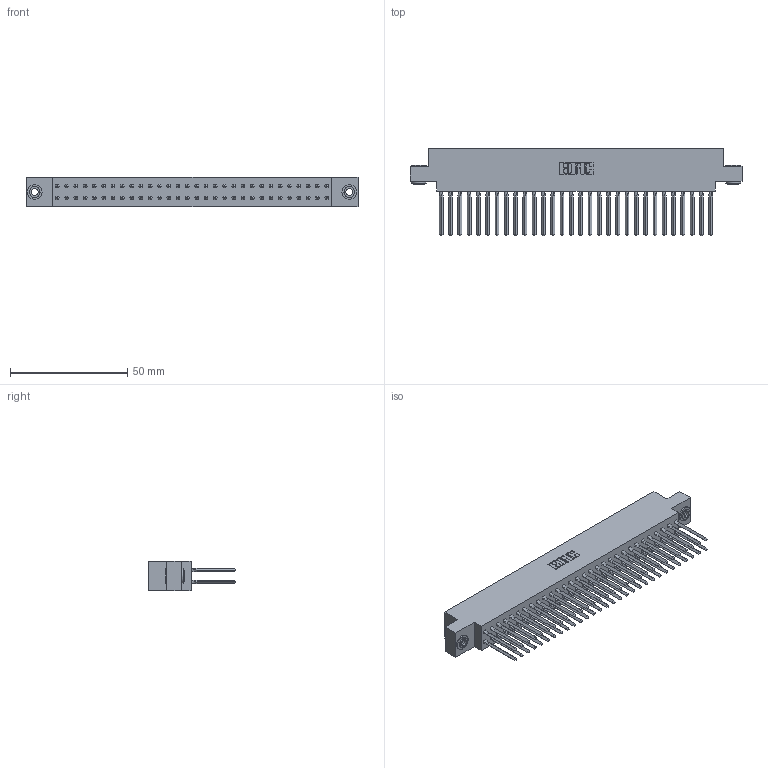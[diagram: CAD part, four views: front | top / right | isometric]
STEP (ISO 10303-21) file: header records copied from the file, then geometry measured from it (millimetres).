
FILE_DESCRIPTION (( 'STEP AP203' ), '1' );
FILE_NAME ('317-060-540-803.STEP', '2020-02-28T04:57:40', ( '' ), ( '' ), 'SwSTEP 2.0', 'SolidWorks 2016', '' );
FILE_SCHEMA (( 'CONFIG_CONTROL_DESIGN' ));
Length unit declared in the file: inch
Products named in the file (4): 317-060-540-803; 345-250-002_345-250-002-102; 317-290-001_540; 317 Part_.156 Dia - TH
Assembly tree (63 placements, depth 2):
  317-060-540-803
    317 Part_.156 Dia - TH
    317-290-001_540  x60
    345-250-002_345-250-002-102  x2
Bounding box: 141.58 x 37.34 x 12.7 mm (x, y, z)
Volume: 23375.1 mm3; surface area: 34610.4 mm2
Topology: 63 solids, 63 shells, 5480 faces, 15171 edges, 9770 vertices
Faces by surface type: plane 4448, cylinder 784, bspline 240, cone 8
Entity records: 45689 total; most frequent: CARTESIAN_POINT 8354, ORIENTED_EDGE 7846, DIRECTION 6587, EDGE_CURVE 3923, LINE 3643, VECTOR 3643, VERTEX_POINT 2607, AXIS2_PLACEMENT_3D 1472
